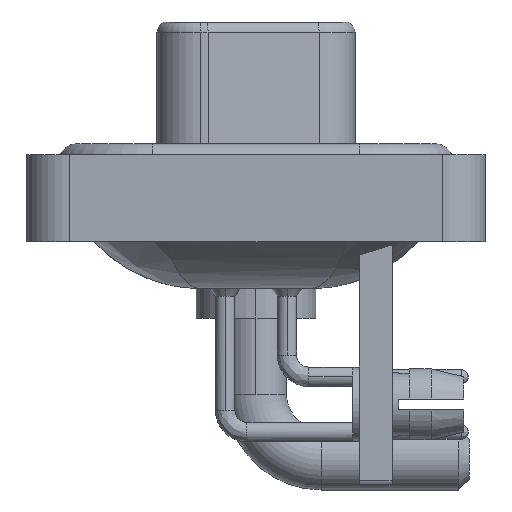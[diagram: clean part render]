
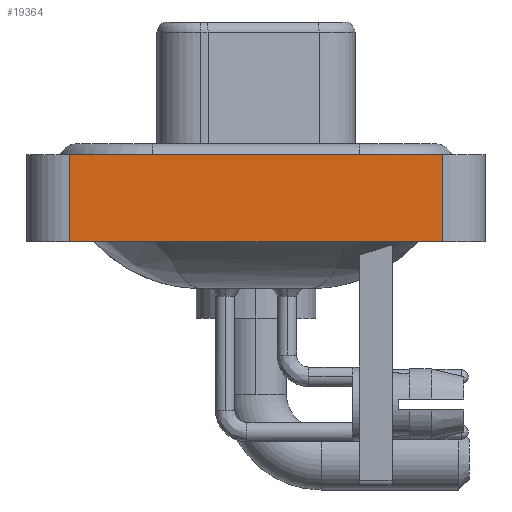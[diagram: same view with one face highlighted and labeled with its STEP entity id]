
A CAD part, left-side view. The second image highlights one B-rep face of the part: STEP entity #19364.
In plain terms, the highlighted planar face has unit normal (-1, 0, 0).
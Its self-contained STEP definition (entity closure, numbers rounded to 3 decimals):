
#231 = ORIENTED_EDGE ( 'NONE', *, *, #16743, .F. ) ;
#1560 = LINE ( 'NONE', #11142, #19283 ) ;
#3409 = CARTESIAN_POINT ( 'NONE',  ( -7.25, 8.55, 0.4 ) ) ;
#3601 = EDGE_CURVE ( 'NONE', #15475, #25133, #14577, .T. ) ;
#4190 = CARTESIAN_POINT ( 'NONE',  ( -7.25, -8.55, -3.6 ) ) ;
#4817 = EDGE_LOOP ( 'NONE', ( #14923, #11409, #231, #18333 ) ) ;
#5970 = CARTESIAN_POINT ( 'NONE',  ( -7.25, -8.55, -3.6 ) ) ;
#7603 = AXIS2_PLACEMENT_3D ( 'NONE', #4190, #8143, #23493 ) ;
#7938 = CARTESIAN_POINT ( 'NONE',  ( -7.25, -8.55, -3.6 ) ) ;
#8143 = DIRECTION ( 'NONE',  ( -1., 0., 0. ) ) ;
#8248 = EDGE_CURVE ( 'NONE', #14654, #25133, #1560, .T. ) ;
#9521 = VECTOR ( 'NONE', #22375, 1000. ) ;
#9931 = DIRECTION ( 'NONE',  ( 0., -1., 0. ) ) ;
#10028 = CARTESIAN_POINT ( 'NONE',  ( -7.25, 8.55, -3.6 ) ) ;
#10193 = FACE_OUTER_BOUND ( 'NONE', #4817, .T. ) ;
#11142 = CARTESIAN_POINT ( 'NONE',  ( -7.25, -8.55, 0.4 ) ) ;
#11409 = ORIENTED_EDGE ( 'NONE', *, *, #8248, .F. ) ;
#11431 = VECTOR ( 'NONE', #9931, 1000. ) ;
#12773 = CARTESIAN_POINT ( 'NONE',  ( -7.25, -8.55, -3.6 ) ) ;
#12785 = DIRECTION ( 'NONE',  ( 0., -1., 0. ) ) ;
#13831 = LINE ( 'NONE', #10028, #19613 ) ;
#14002 = CARTESIAN_POINT ( 'NONE',  ( -7.25, -8.55, 0.4 ) ) ;
#14577 = LINE ( 'NONE', #12773, #9521 ) ;
#14654 = VERTEX_POINT ( 'NONE', #3409 ) ;
#14923 = ORIENTED_EDGE ( 'NONE', *, *, #3601, .T. ) ;
#15475 = VERTEX_POINT ( 'NONE', #7938 ) ;
#15811 = PLANE ( 'NONE',  #7603 ) ;
#16743 = EDGE_CURVE ( 'NONE', #25014, #14654, #13831, .T. ) ;
#17517 = EDGE_CURVE ( 'NONE', #25014, #15475, #19628, .T. ) ;
#18333 = ORIENTED_EDGE ( 'NONE', *, *, #17517, .T. ) ;
#19283 = VECTOR ( 'NONE', #12785, 1000. ) ;
#19364 = ADVANCED_FACE ( 'NONE', ( #10193 ), #15811, .T. ) ;
#19510 = CARTESIAN_POINT ( 'NONE',  ( -7.25, 8.55, -3.6 ) ) ;
#19613 = VECTOR ( 'NONE', #23681, 1000. ) ;
#19628 = LINE ( 'NONE', #5970, #11431 ) ;
#22375 = DIRECTION ( 'NONE',  ( 0., 0., 1. ) ) ;
#23493 = DIRECTION ( 'NONE',  ( 0., 0., 1. ) ) ;
#23681 = DIRECTION ( 'NONE',  ( 0., 0., 1. ) ) ;
#25014 = VERTEX_POINT ( 'NONE', #19510 ) ;
#25133 = VERTEX_POINT ( 'NONE', #14002 ) ;
